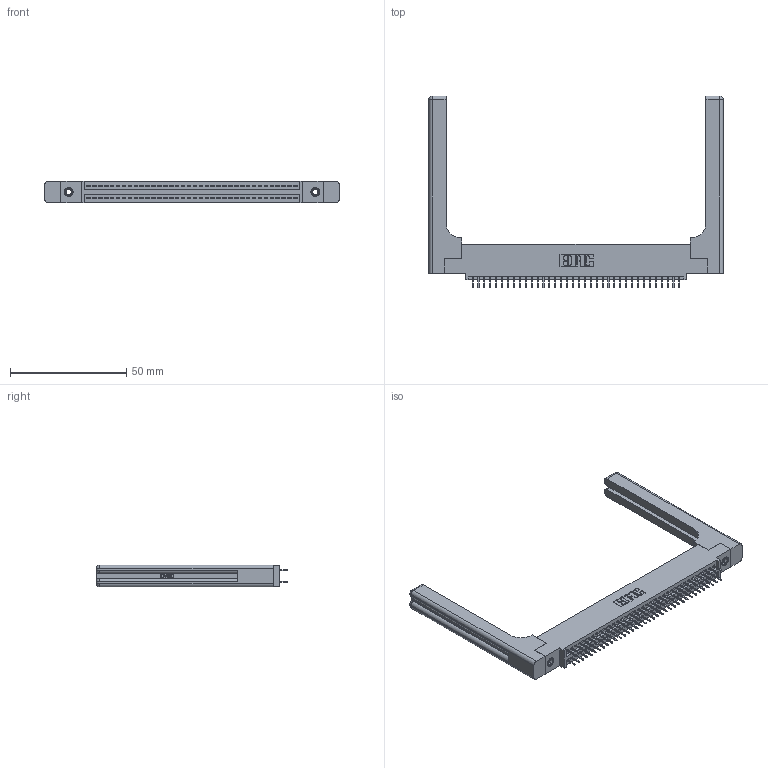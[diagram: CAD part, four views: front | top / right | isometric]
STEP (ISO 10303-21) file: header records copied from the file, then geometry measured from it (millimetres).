
FILE_DESCRIPTION (( 'STEP AP203' ), '1' );
FILE_NAME ('395-072-525-558.STEP', '2020-09-25T07:49:59', ( '' ), ( '' ), 'SwSTEP 2.0', 'SolidWorks 2020', '' );
FILE_SCHEMA (( 'CONFIG_CONTROL_DESIGN' ));
Length unit declared in the file: inch
Products named in the file (5): 345-292-001_345-293-125; 395-072-525-558; 345-250-001_345-250-001-102; 345-220-058_345-220-058; 345 Part_0.110 Offset - 0.156 Dia-TH
Assembly tree (77 placements, depth 2):
  395-072-525-558
    345 Part_0.110 Offset - 0.156 Dia-TH
    345-292-001_345-293-125  x72
    345-250-001_345-250-001-102  x2
    345-220-058_345-220-058  x2
Bounding box: 126.47 x 82.47 x 9.4 mm (x, y, z)
Volume: 20512.6 mm3; surface area: 22471.8 mm2
Topology: 77 solids, 77 shells, 4274 faces, 12035 edges, 7714 vertices
Faces by surface type: plane 3040, cylinder 1174, bspline 36, cone 12, sphere 8, torus 4
Entity records: 34442 total; most frequent: CARTESIAN_POINT 6773, ORIENTED_EDGE 5504, DIRECTION 4912, EDGE_CURVE 2752, LINE 2388, VECTOR 2388, VERTEX_POINT 1822, AXIS2_PLACEMENT_3D 1262
